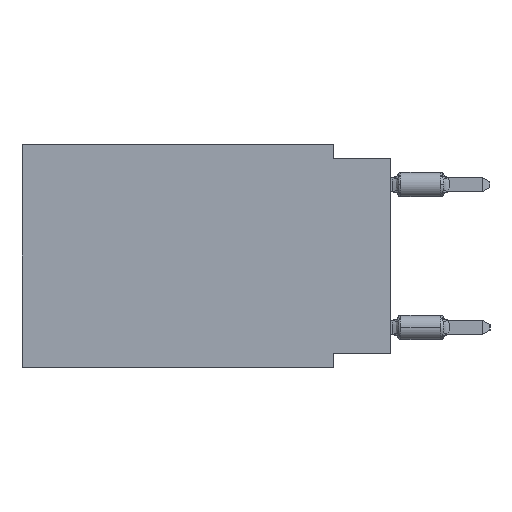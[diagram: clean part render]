
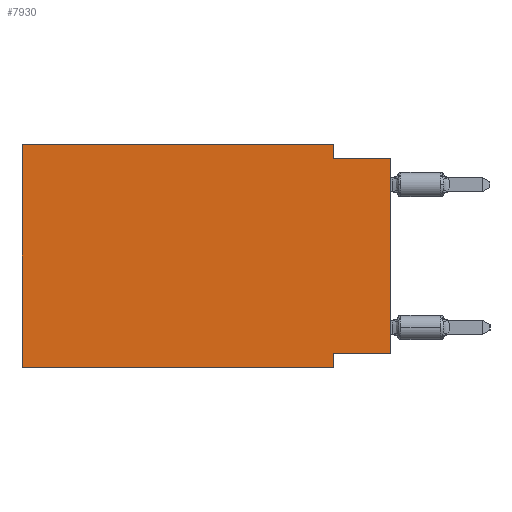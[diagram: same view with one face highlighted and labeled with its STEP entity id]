
A CAD part, left-side view. The second image highlights one B-rep face of the part: STEP entity #7930.
In plain terms, the highlighted planar face has unit normal (-1, 0, 0).
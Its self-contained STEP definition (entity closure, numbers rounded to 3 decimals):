
#447 = VERTEX_POINT ( 'NONE', #12749 ) ;
#713 = CARTESIAN_POINT ( 'NONE',  ( 0., 16.383, -9.906 ) ) ;
#836 = LINE ( 'NONE', #15331, #4758 ) ;
#1133 = EDGE_LOOP ( 'NONE', ( #3293, #27739, #12728, #1851, #4202, #14385, #3183, #8335 ) ) ;
#1230 = LINE ( 'NONE', #20283, #7057 ) ;
#1422 = DIRECTION ( 'NONE',  ( 1., 0., 0. ) ) ;
#1798 = LINE ( 'NONE', #23720, #10530 ) ;
#1851 = ORIENTED_EDGE ( 'NONE', *, *, #8663, .F. ) ;
#3183 = ORIENTED_EDGE ( 'NONE', *, *, #29849, .F. ) ;
#3293 = ORIENTED_EDGE ( 'NONE', *, *, #4470, .T. ) ;
#3725 = LINE ( 'NONE', #20117, #8108 ) ;
#4202 = ORIENTED_EDGE ( 'NONE', *, *, #23306, .F. ) ;
#4470 = EDGE_CURVE ( 'NONE', #25888, #26786, #3725, .T. ) ;
#4709 = AXIS2_PLACEMENT_3D ( 'NONE', #8829, #1422, #25405 ) ;
#4758 = VECTOR ( 'NONE', #5872, 1000. ) ;
#5872 = DIRECTION ( 'NONE',  ( 0., -1., 0. ) ) ;
#6064 = LINE ( 'NONE', #713, #30942 ) ;
#7057 = VECTOR ( 'NONE', #30095, 1000. ) ;
#7930 = ADVANCED_FACE ( 'NONE', ( #20326 ), #22865, .F. ) ;
#8108 = VECTOR ( 'NONE', #11569, 1000. ) ;
#8202 = DIRECTION ( 'NONE',  ( 0., 0., -1. ) ) ;
#8335 = ORIENTED_EDGE ( 'NONE', *, *, #19273, .F. ) ;
#8663 = EDGE_CURVE ( 'NONE', #13111, #17326, #836, .T. ) ;
#8829 = CARTESIAN_POINT ( 'NONE',  ( 0., 16.383, 0. ) ) ;
#9289 = VECTOR ( 'NONE', #8202, 1000. ) ;
#10530 = VECTOR ( 'NONE', #28452, 1000. ) ;
#10893 = LINE ( 'NONE', #20493, #9289 ) ;
#11235 = VECTOR ( 'NONE', #27472, 1000. ) ;
#11268 = CARTESIAN_POINT ( 'NONE',  ( 0., 2.54, -0.635 ) ) ;
#11569 = DIRECTION ( 'NONE',  ( 0., 0., 1. ) ) ;
#11589 = EDGE_CURVE ( 'NONE', #29385, #11950, #6064, .T. ) ;
#11728 = VERTEX_POINT ( 'NONE', #11268 ) ;
#11950 = VERTEX_POINT ( 'NONE', #30022 ) ;
#12728 = ORIENTED_EDGE ( 'NONE', *, *, #13668, .F. ) ;
#12749 = CARTESIAN_POINT ( 'NONE',  ( 0., 2.54, -9.271 ) ) ;
#13111 = VERTEX_POINT ( 'NONE', #22120 ) ;
#13668 = EDGE_CURVE ( 'NONE', #17326, #11728, #10893, .T. ) ;
#14385 = ORIENTED_EDGE ( 'NONE', *, *, #11589, .T. ) ;
#15331 = CARTESIAN_POINT ( 'NONE',  ( 0., 16.383, 0. ) ) ;
#15499 = CARTESIAN_POINT ( 'NONE',  ( 0., 16.383, -9.906 ) ) ;
#17326 = VERTEX_POINT ( 'NONE', #24258 ) ;
#17489 = CARTESIAN_POINT ( 'NONE',  ( 0., 2.54, -9.906 ) ) ;
#17799 = LINE ( 'NONE', #17489, #11235 ) ;
#18058 = EDGE_CURVE ( 'NONE', #11728, #26786, #1798, .T. ) ;
#19273 = EDGE_CURVE ( 'NONE', #25888, #447, #1230, .T. ) ;
#20117 = CARTESIAN_POINT ( 'NONE',  ( 0., 0., 0. ) ) ;
#20283 = CARTESIAN_POINT ( 'NONE',  ( 0., 0., -9.271 ) ) ;
#20326 = FACE_OUTER_BOUND ( 'NONE', #1133, .T. ) ;
#20493 = CARTESIAN_POINT ( 'NONE',  ( 0., 2.54, 0. ) ) ;
#22120 = CARTESIAN_POINT ( 'NONE',  ( 0., 16.383, 0. ) ) ;
#22404 = LINE ( 'NONE', #26994, #27874 ) ;
#22865 = PLANE ( 'NONE',  #4709 ) ;
#23306 = EDGE_CURVE ( 'NONE', #29385, #13111, #22404, .T. ) ;
#23720 = CARTESIAN_POINT ( 'NONE',  ( 0., 0., -0.635 ) ) ;
#24258 = CARTESIAN_POINT ( 'NONE',  ( 0., 2.54, 0. ) ) ;
#24696 = DIRECTION ( 'NONE',  ( 0., -1., 0. ) ) ;
#25098 = DIRECTION ( 'NONE',  ( 0., 0., 1. ) ) ;
#25405 = DIRECTION ( 'NONE',  ( 0., 0., -1. ) ) ;
#25888 = VERTEX_POINT ( 'NONE', #26039 ) ;
#25952 = CARTESIAN_POINT ( 'NONE',  ( 0., 0., -0.635 ) ) ;
#26039 = CARTESIAN_POINT ( 'NONE',  ( 0., 0., -9.271 ) ) ;
#26786 = VERTEX_POINT ( 'NONE', #25952 ) ;
#26994 = CARTESIAN_POINT ( 'NONE',  ( 0., 16.383, 0. ) ) ;
#27472 = DIRECTION ( 'NONE',  ( 0., 0., -1. ) ) ;
#27739 = ORIENTED_EDGE ( 'NONE', *, *, #18058, .F. ) ;
#27874 = VECTOR ( 'NONE', #25098, 1000. ) ;
#28452 = DIRECTION ( 'NONE',  ( 0., -1., 0. ) ) ;
#29385 = VERTEX_POINT ( 'NONE', #15499 ) ;
#29849 = EDGE_CURVE ( 'NONE', #447, #11950, #17799, .T. ) ;
#30022 = CARTESIAN_POINT ( 'NONE',  ( 0., 2.54, -9.906 ) ) ;
#30095 = DIRECTION ( 'NONE',  ( 0., 1., 0. ) ) ;
#30942 = VECTOR ( 'NONE', #24696, 1000. ) ;
